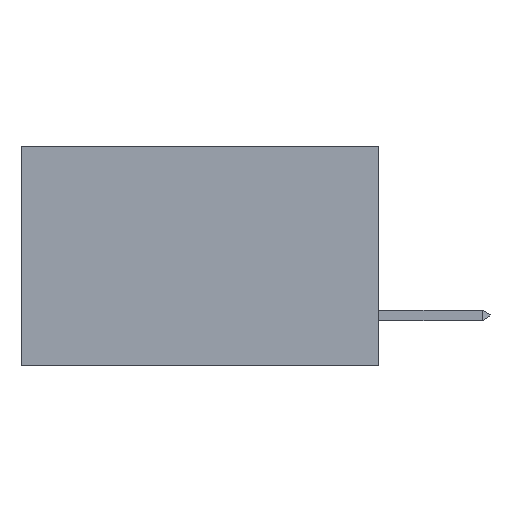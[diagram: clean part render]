
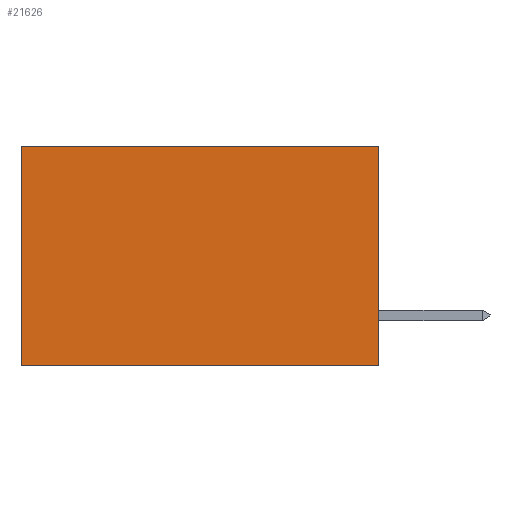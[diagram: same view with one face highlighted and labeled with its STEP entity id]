
A CAD part, left-side view. The second image highlights one B-rep face of the part: STEP entity #21626.
In plain terms, the highlighted planar face has unit normal (-1, 0, 0).
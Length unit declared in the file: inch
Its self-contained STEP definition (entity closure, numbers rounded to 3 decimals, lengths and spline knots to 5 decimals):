
#93 = DIRECTION ( 'NONE',  ( 0., 1., 0. ) ) ;
#1323 = CARTESIAN_POINT ( 'NONE',  ( 0.298, 0., -0.37 ) ) ;
#1571 = VERTEX_POINT ( 'NONE', #20209 ) ;
#1830 = EDGE_CURVE ( 'NONE', #1571, #9995, #15491, .T. ) ;
#2164 = DIRECTION ( 'NONE',  ( 0., 0., -1. ) ) ;
#2887 = VECTOR ( 'NONE', #2164, 39.37008 ) ;
#3125 = CARTESIAN_POINT ( 'NONE',  ( 0.298, 0., 0. ) ) ;
#3155 = LINE ( 'NONE', #5658, #6138 ) ;
#4078 = ORIENTED_EDGE ( 'NONE', *, *, #18194, .T. ) ;
#4183 = LINE ( 'NONE', #17363, #9647 ) ;
#5078 = PLANE ( 'NONE',  #6662 ) ;
#5658 = CARTESIAN_POINT ( 'NONE',  ( 0.298, 0., -0.37 ) ) ;
#6138 = VECTOR ( 'NONE', #19108, 39.37008 ) ;
#6249 = CARTESIAN_POINT ( 'NONE',  ( 0.298, 0.6, -0.37 ) ) ;
#6559 = DIRECTION ( 'NONE',  ( 0., 0., -1. ) ) ;
#6662 = AXIS2_PLACEMENT_3D ( 'NONE', #24063, #6741, #20376 ) ;
#6708 = VECTOR ( 'NONE', #6559, 39.37008 ) ;
#6741 = DIRECTION ( 'NONE',  ( 1., 0., 0. ) ) ;
#8799 = VERTEX_POINT ( 'NONE', #20022 ) ;
#9363 = ORIENTED_EDGE ( 'NONE', *, *, #1830, .F. ) ;
#9647 = VECTOR ( 'NONE', #93, 39.37008 ) ;
#9995 = VERTEX_POINT ( 'NONE', #1323 ) ;
#11036 = EDGE_CURVE ( 'NONE', #9995, #15044, #3155, .T. ) ;
#13181 = LINE ( 'NONE', #19181, #2887 ) ;
#15044 = VERTEX_POINT ( 'NONE', #6249 ) ;
#15491 = LINE ( 'NONE', #3125, #6708 ) ;
#17363 = CARTESIAN_POINT ( 'NONE',  ( 0.298, 0., 0. ) ) ;
#18194 = EDGE_CURVE ( 'NONE', #8799, #15044, #13181, .T. ) ;
#19108 = DIRECTION ( 'NONE',  ( 0., 1., 0. ) ) ;
#19181 = CARTESIAN_POINT ( 'NONE',  ( 0.298, 0.6, 0. ) ) ;
#19523 = ORIENTED_EDGE ( 'NONE', *, *, #11036, .F. ) ;
#20022 = CARTESIAN_POINT ( 'NONE',  ( 0.298, 0.6, 0. ) ) ;
#20209 = CARTESIAN_POINT ( 'NONE',  ( 0.298, 0., 0. ) ) ;
#20376 = DIRECTION ( 'NONE',  ( 0., 0., -1. ) ) ;
#21626 = ADVANCED_FACE ( 'NONE', ( #22407 ), #5078, .F. ) ;
#22037 = ORIENTED_EDGE ( 'NONE', *, *, #23338, .T. ) ;
#22407 = FACE_OUTER_BOUND ( 'NONE', #24290, .T. ) ;
#23338 = EDGE_CURVE ( 'NONE', #1571, #8799, #4183, .T. ) ;
#24063 = CARTESIAN_POINT ( 'NONE',  ( 0.298, 0., 0. ) ) ;
#24290 = EDGE_LOOP ( 'NONE', ( #4078, #19523, #9363, #22037 ) ) ;
